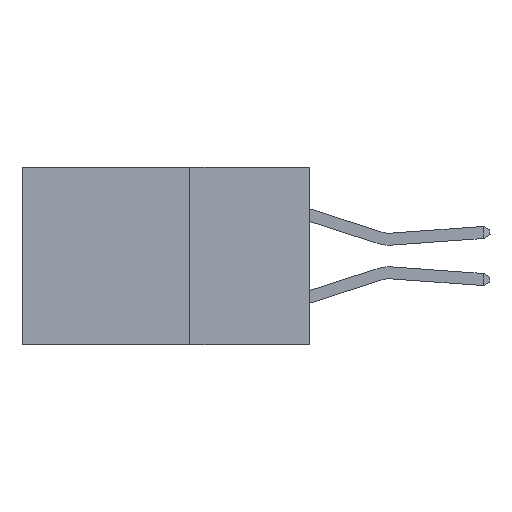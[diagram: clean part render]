
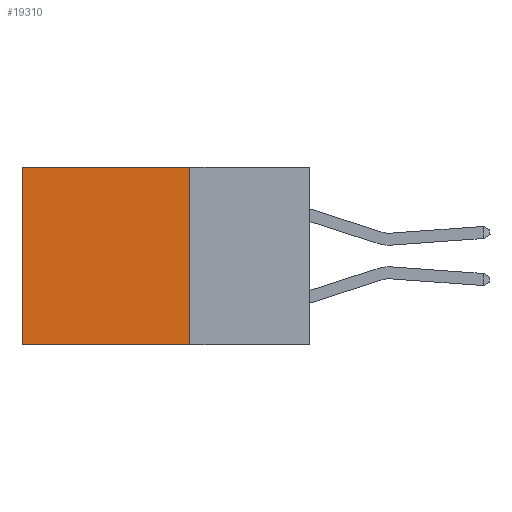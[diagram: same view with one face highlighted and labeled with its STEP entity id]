
A CAD part, left-side view. The second image highlights one B-rep face of the part: STEP entity #19310.
In plain terms, the highlighted planar face has unit normal (-1, 0, 0).
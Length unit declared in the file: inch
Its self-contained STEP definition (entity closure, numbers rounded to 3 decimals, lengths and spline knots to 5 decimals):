
#527 = VECTOR ( 'NONE', #18451, 39.37008 ) ;
#760 = PLANE ( 'NONE',  #3986 ) ;
#902 = VERTEX_POINT ( 'NONE', #14721 ) ;
#1778 = CARTESIAN_POINT ( 'NONE',  ( 0.2615, 0.25, 0. ) ) ;
#2955 = CARTESIAN_POINT ( 'NONE',  ( 0.2615, 0.25, 0. ) ) ;
#3167 = VECTOR ( 'NONE', #7676, 39.37008 ) ;
#3621 = EDGE_CURVE ( 'NONE', #6277, #902, #12251, .T. ) ;
#3986 = AXIS2_PLACEMENT_3D ( 'NONE', #13231, #7869, #9615 ) ;
#6277 = VERTEX_POINT ( 'NONE', #13213 ) ;
#7676 = DIRECTION ( 'NONE',  ( 0., 1., 0. ) ) ;
#7869 = DIRECTION ( 'NONE',  ( 1., 0., 0. ) ) ;
#8265 = VERTEX_POINT ( 'NONE', #15741 ) ;
#8618 = DIRECTION ( 'NONE',  ( 0., 0., -1. ) ) ;
#9306 = VECTOR ( 'NONE', #8618, 39.37008 ) ;
#9615 = DIRECTION ( 'NONE',  ( 0., 0., -1. ) ) ;
#9810 = LINE ( 'NONE', #20198, #527 ) ;
#12251 = LINE ( 'NONE', #22635, #9306 ) ;
#13213 = CARTESIAN_POINT ( 'NONE',  ( 0.2615, 0.6, 0. ) ) ;
#13231 = CARTESIAN_POINT ( 'NONE',  ( 0.2615, 0.25, -0.37 ) ) ;
#13701 = EDGE_CURVE ( 'NONE', #14581, #8265, #9810, .T. ) ;
#14231 = LINE ( 'NONE', #21234, #3167 ) ;
#14581 = VERTEX_POINT ( 'NONE', #2955 ) ;
#14599 = ORIENTED_EDGE ( 'NONE', *, *, #3621, .T. ) ;
#14721 = CARTESIAN_POINT ( 'NONE',  ( 0.2615, 0.6, -0.37 ) ) ;
#15741 = CARTESIAN_POINT ( 'NONE',  ( 0.2615, 0.25, -0.37 ) ) ;
#16018 = LINE ( 'NONE', #1778, #19266 ) ;
#16963 = ORIENTED_EDGE ( 'NONE', *, *, #19562, .T. ) ;
#17006 = EDGE_CURVE ( 'NONE', #8265, #902, #14231, .T. ) ;
#17529 = DIRECTION ( 'NONE',  ( 0., 1., 0. ) ) ;
#18371 = FACE_OUTER_BOUND ( 'NONE', #21843, .T. ) ;
#18451 = DIRECTION ( 'NONE',  ( 0., 0., -1. ) ) ;
#18981 = ORIENTED_EDGE ( 'NONE', *, *, #13701, .F. ) ;
#19266 = VECTOR ( 'NONE', #17529, 39.37008 ) ;
#19310 = ADVANCED_FACE ( 'NONE', ( #18371 ), #760, .F. ) ;
#19562 = EDGE_CURVE ( 'NONE', #14581, #6277, #16018, .T. ) ;
#20142 = ORIENTED_EDGE ( 'NONE', *, *, #17006, .F. ) ;
#20198 = CARTESIAN_POINT ( 'NONE',  ( 0.2615, 0.25, -0.37 ) ) ;
#21234 = CARTESIAN_POINT ( 'NONE',  ( 0.2615, 0.25, -0.37 ) ) ;
#21843 = EDGE_LOOP ( 'NONE', ( #14599, #20142, #18981, #16963 ) ) ;
#22635 = CARTESIAN_POINT ( 'NONE',  ( 0.2615, 0.6, -0.37 ) ) ;
